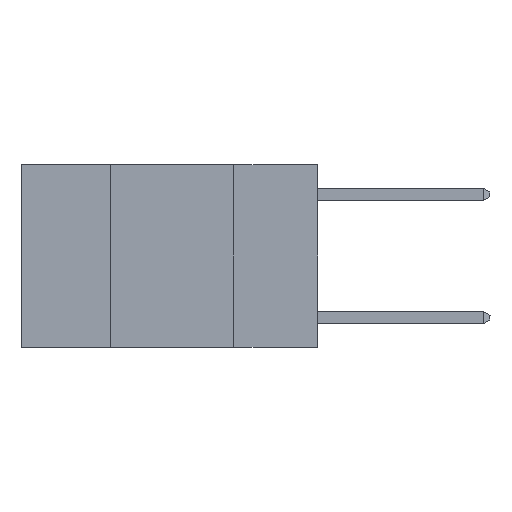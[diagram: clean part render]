
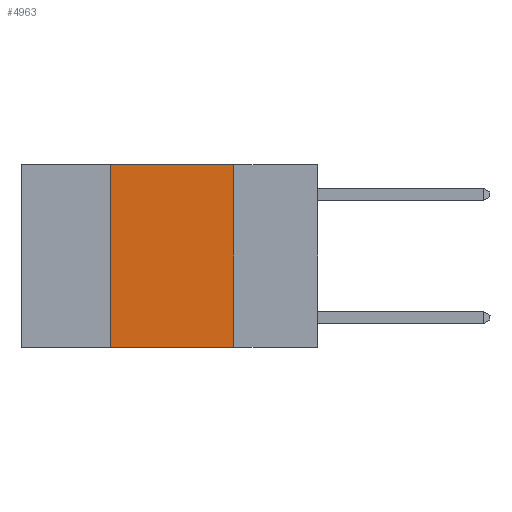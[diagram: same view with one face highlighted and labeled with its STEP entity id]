
A CAD part, left-side view. The second image highlights one B-rep face of the part: STEP entity #4963.
In plain terms, the highlighted planar face has unit normal (-1, 0, 0).
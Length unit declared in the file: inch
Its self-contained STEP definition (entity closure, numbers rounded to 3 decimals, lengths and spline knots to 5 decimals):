
#248 = CARTESIAN_POINT ( 'NONE',  ( 0., 0.17, 0. ) ) ;
#2279 = DIRECTION ( 'NONE',  ( 0., -1., 0. ) ) ;
#3173 = CARTESIAN_POINT ( 'NONE',  ( 0., 0.17, -0.37 ) ) ;
#4963 = ADVANCED_FACE ( 'NONE', ( #21551 ), #27894, .F. ) ;
#5716 = VECTOR ( 'NONE', #20621, 39.37008 ) ;
#7176 = EDGE_CURVE ( 'NONE', #20420, #15956, #23823, .T. ) ;
#8994 = ORIENTED_EDGE ( 'NONE', *, *, #12340, .F. ) ;
#9203 = AXIS2_PLACEMENT_3D ( 'NONE', #10060, #25735, #12336 ) ;
#9783 = ORIENTED_EDGE ( 'NONE', *, *, #24798, .F. ) ;
#9998 = ORIENTED_EDGE ( 'NONE', *, *, #20555, .F. ) ;
#10060 = CARTESIAN_POINT ( 'NONE',  ( 0., 0.6, 0. ) ) ;
#10515 = EDGE_LOOP ( 'NONE', ( #8994, #9783, #9998, #10625 ) ) ;
#10625 = ORIENTED_EDGE ( 'NONE', *, *, #7176, .T. ) ;
#11357 = CARTESIAN_POINT ( 'NONE',  ( 0., 0.42, -0.37 ) ) ;
#11918 = VECTOR ( 'NONE', #24711, 39.37008 ) ;
#12336 = DIRECTION ( 'NONE',  ( 0., 0., -1. ) ) ;
#12340 = EDGE_CURVE ( 'NONE', #14510, #15956, #28883, .T. ) ;
#13534 = CARTESIAN_POINT ( 'NONE',  ( 0., 0.42, 0. ) ) ;
#14510 = VERTEX_POINT ( 'NONE', #23529 ) ;
#14921 = VERTEX_POINT ( 'NONE', #13534 ) ;
#15956 = VERTEX_POINT ( 'NONE', #3173 ) ;
#18084 = CARTESIAN_POINT ( 'NONE',  ( 0., 0.6, 0. ) ) ;
#19212 = LINE ( 'NONE', #25342, #24413 ) ;
#20420 = VERTEX_POINT ( 'NONE', #11357 ) ;
#20555 = EDGE_CURVE ( 'NONE', #20420, #14921, #19212, .T. ) ;
#20621 = DIRECTION ( 'NONE',  ( 0., 0., -1. ) ) ;
#21551 = FACE_OUTER_BOUND ( 'NONE', #10515, .T. ) ;
#22024 = LINE ( 'NONE', #18084, #22698 ) ;
#22478 = CARTESIAN_POINT ( 'NONE',  ( 0., 0.6, -0.37 ) ) ;
#22698 = VECTOR ( 'NONE', #2279, 39.37008 ) ;
#23529 = CARTESIAN_POINT ( 'NONE',  ( 0., 0.17, 0. ) ) ;
#23823 = LINE ( 'NONE', #22478, #11918 ) ;
#24413 = VECTOR ( 'NONE', #27590, 39.37008 ) ;
#24711 = DIRECTION ( 'NONE',  ( 0., -1., 0. ) ) ;
#24798 = EDGE_CURVE ( 'NONE', #14921, #14510, #22024, .T. ) ;
#25342 = CARTESIAN_POINT ( 'NONE',  ( 0., 0.42, 0. ) ) ;
#25735 = DIRECTION ( 'NONE',  ( 1., 0., 0. ) ) ;
#27590 = DIRECTION ( 'NONE',  ( 0., 0., 1. ) ) ;
#27894 = PLANE ( 'NONE',  #9203 ) ;
#28883 = LINE ( 'NONE', #248, #5716 ) ;
